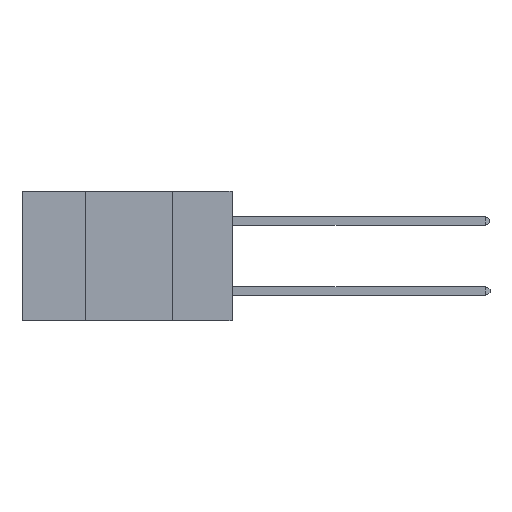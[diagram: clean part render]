
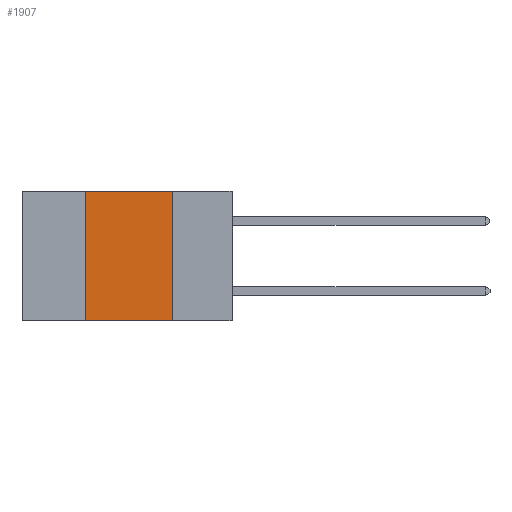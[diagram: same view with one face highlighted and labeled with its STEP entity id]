
A CAD part, left-side view. The second image highlights one B-rep face of the part: STEP entity #1907.
In plain terms, the highlighted planar face has unit normal (-1, 0, 0).
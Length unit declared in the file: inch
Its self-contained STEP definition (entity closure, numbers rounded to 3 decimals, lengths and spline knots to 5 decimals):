
#273 = CARTESIAN_POINT ( 'NONE',  ( 0., 0.17, -0.37 ) ) ;
#407 = EDGE_CURVE ( 'NONE', #1639, #13925, #13549, .T. ) ;
#467 = CARTESIAN_POINT ( 'NONE',  ( 0., 0.6, 0. ) ) ;
#916 = VECTOR ( 'NONE', #8034, 39.37008 ) ;
#1549 = LINE ( 'NONE', #2450, #916 ) ;
#1596 = CARTESIAN_POINT ( 'NONE',  ( 0., 0.17, 0. ) ) ;
#1639 = VERTEX_POINT ( 'NONE', #21032 ) ;
#1907 = ADVANCED_FACE ( 'NONE', ( #11533 ), #9626, .F. ) ;
#2258 = CARTESIAN_POINT ( 'NONE',  ( 0., 0.6, 0. ) ) ;
#2450 = CARTESIAN_POINT ( 'NONE',  ( 0., 0.6, -0.37 ) ) ;
#4368 = DIRECTION ( 'NONE',  ( 0., -1., 0. ) ) ;
#5578 = EDGE_CURVE ( 'NONE', #1639, #11118, #1549, .T. ) ;
#6074 = AXIS2_PLACEMENT_3D ( 'NONE', #2258, #6094, #18639 ) ;
#6094 = DIRECTION ( 'NONE',  ( 1., 0., 0. ) ) ;
#7241 = DIRECTION ( 'NONE',  ( 0., 0., -1. ) ) ;
#7841 = CARTESIAN_POINT ( 'NONE',  ( 0., 0.17, 0. ) ) ;
#8034 = DIRECTION ( 'NONE',  ( 0., -1., 0. ) ) ;
#8124 = VECTOR ( 'NONE', #4368, 39.37008 ) ;
#8657 = VECTOR ( 'NONE', #7241, 39.37008 ) ;
#9626 = PLANE ( 'NONE',  #6074 ) ;
#10501 = ORIENTED_EDGE ( 'NONE', *, *, #14496, .F. ) ;
#11118 = VERTEX_POINT ( 'NONE', #273 ) ;
#11533 = FACE_OUTER_BOUND ( 'NONE', #18511, .T. ) ;
#11647 = DIRECTION ( 'NONE',  ( 0., 0., 1. ) ) ;
#12551 = CARTESIAN_POINT ( 'NONE',  ( 0., 0.42, 0. ) ) ;
#12971 = VECTOR ( 'NONE', #11647, 39.37008 ) ;
#13549 = LINE ( 'NONE', #12551, #12971 ) ;
#13925 = VERTEX_POINT ( 'NONE', #23445 ) ;
#14496 = EDGE_CURVE ( 'NONE', #22844, #11118, #22935, .T. ) ;
#17957 = ORIENTED_EDGE ( 'NONE', *, *, #5578, .T. ) ;
#18511 = EDGE_LOOP ( 'NONE', ( #10501, #21492, #20987, #17957 ) ) ;
#18639 = DIRECTION ( 'NONE',  ( 0., 0., -1. ) ) ;
#20987 = ORIENTED_EDGE ( 'NONE', *, *, #407, .F. ) ;
#21032 = CARTESIAN_POINT ( 'NONE',  ( 0., 0.42, -0.37 ) ) ;
#21492 = ORIENTED_EDGE ( 'NONE', *, *, #22258, .F. ) ;
#22258 = EDGE_CURVE ( 'NONE', #13925, #22844, #22416, .T. ) ;
#22416 = LINE ( 'NONE', #467, #8124 ) ;
#22844 = VERTEX_POINT ( 'NONE', #7841 ) ;
#22935 = LINE ( 'NONE', #1596, #8657 ) ;
#23445 = CARTESIAN_POINT ( 'NONE',  ( 0., 0.42, 0. ) ) ;
